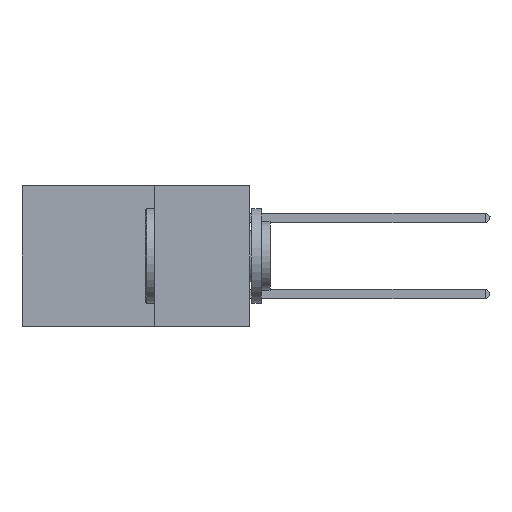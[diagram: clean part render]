
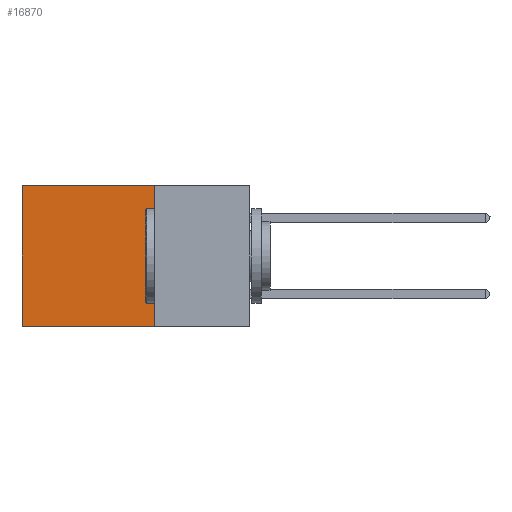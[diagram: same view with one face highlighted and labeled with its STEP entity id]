
A CAD part, left-side view. The second image highlights one B-rep face of the part: STEP entity #16870.
In plain terms, the highlighted planar face has unit normal (-1, 0, 0).
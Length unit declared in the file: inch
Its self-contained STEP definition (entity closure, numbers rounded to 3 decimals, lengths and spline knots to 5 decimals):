
#285 = VECTOR ( 'NONE', #3150, 39.37008 ) ;
#3150 = DIRECTION ( 'NONE',  ( 0., 0., -1. ) ) ;
#4511 = CARTESIAN_POINT ( 'NONE',  ( 0.2875, 0.25, 0. ) ) ;
#6991 = PLANE ( 'NONE',  #15496 ) ;
#8076 = VECTOR ( 'NONE', #32435, 39.37008 ) ;
#8117 = DIRECTION ( 'NONE',  ( 0., 1., 0. ) ) ;
#9390 = EDGE_CURVE ( 'NONE', #39194, #17594, #18143, .T. ) ;
#10007 = ORIENTED_EDGE ( 'NONE', *, *, #9390, .T. ) ;
#11601 = CARTESIAN_POINT ( 'NONE',  ( 0.2875, 0.6, -0.37 ) ) ;
#13357 = VECTOR ( 'NONE', #8117, 39.37008 ) ;
#15496 = AXIS2_PLACEMENT_3D ( 'NONE', #24608, #21207, #45982 ) ;
#16870 = ADVANCED_FACE ( 'NONE', ( #21203 ), #6991, .F. ) ;
#17488 = LINE ( 'NONE', #32581, #8076 ) ;
#17594 = VERTEX_POINT ( 'NONE', #11601 ) ;
#18143 = LINE ( 'NONE', #24391, #285 ) ;
#19172 = EDGE_LOOP ( 'NONE', ( #10007, #34529, #41781, #32966 ) ) ;
#19806 = CARTESIAN_POINT ( 'NONE',  ( 0.2875, 0.25, 0. ) ) ;
#20697 = CARTESIAN_POINT ( 'NONE',  ( 0.2875, 0.6, 0. ) ) ;
#21203 = FACE_OUTER_BOUND ( 'NONE', #19172, .T. ) ;
#21207 = DIRECTION ( 'NONE',  ( 1., 0., 0. ) ) ;
#24391 = CARTESIAN_POINT ( 'NONE',  ( 0.2875, 0.6, 0. ) ) ;
#24608 = CARTESIAN_POINT ( 'NONE',  ( 0.2875, 0.25, 0. ) ) ;
#29707 = EDGE_CURVE ( 'NONE', #37886, #39194, #41520, .T. ) ;
#32435 = DIRECTION ( 'NONE',  ( 0., 0., -1. ) ) ;
#32581 = CARTESIAN_POINT ( 'NONE',  ( 0.2875, 0.25, 0. ) ) ;
#32943 = LINE ( 'NONE', #34484, #40124 ) ;
#32966 = ORIENTED_EDGE ( 'NONE', *, *, #29707, .T. ) ;
#34028 = VERTEX_POINT ( 'NONE', #37160 ) ;
#34484 = CARTESIAN_POINT ( 'NONE',  ( 0.2875, 0.25, -0.37 ) ) ;
#34529 = ORIENTED_EDGE ( 'NONE', *, *, #43768, .F. ) ;
#37160 = CARTESIAN_POINT ( 'NONE',  ( 0.2875, 0.25, -0.37 ) ) ;
#37886 = VERTEX_POINT ( 'NONE', #19806 ) ;
#38048 = DIRECTION ( 'NONE',  ( 0., 1., 0. ) ) ;
#39194 = VERTEX_POINT ( 'NONE', #20697 ) ;
#40124 = VECTOR ( 'NONE', #38048, 39.37008 ) ;
#41520 = LINE ( 'NONE', #4511, #13357 ) ;
#41781 = ORIENTED_EDGE ( 'NONE', *, *, #44102, .F. ) ;
#43768 = EDGE_CURVE ( 'NONE', #34028, #17594, #32943, .T. ) ;
#44102 = EDGE_CURVE ( 'NONE', #37886, #34028, #17488, .T. ) ;
#45982 = DIRECTION ( 'NONE',  ( 0., 0., -1. ) ) ;
